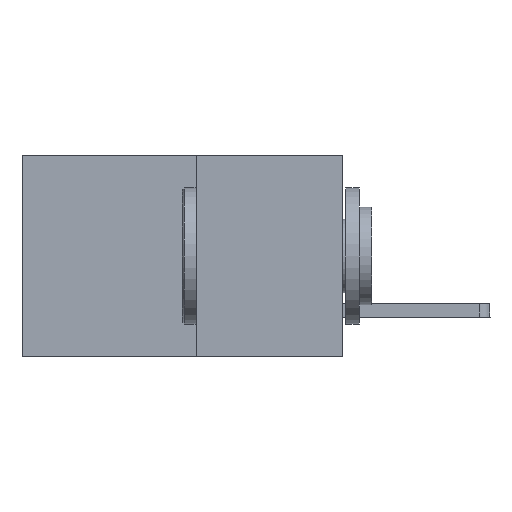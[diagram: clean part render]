
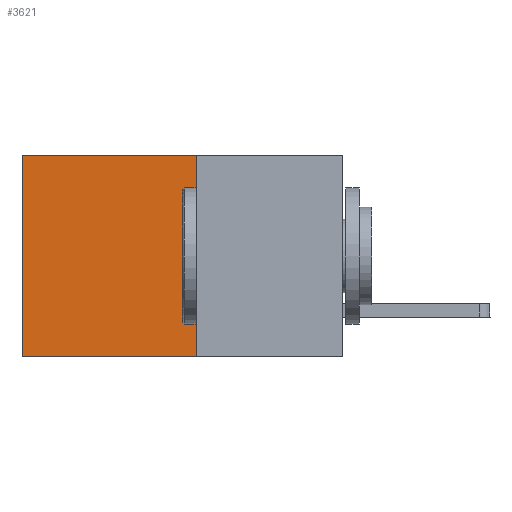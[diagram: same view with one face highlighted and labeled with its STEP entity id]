
A CAD part, left-side view. The second image highlights one B-rep face of the part: STEP entity #3621.
In plain terms, the highlighted planar face has unit normal (-1, 0, 0).
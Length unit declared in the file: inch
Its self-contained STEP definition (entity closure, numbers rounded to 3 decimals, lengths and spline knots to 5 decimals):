
#257 = AXIS2_PLACEMENT_3D ( 'NONE', #3014, #3923, #6539 ) ;
#1044 = DIRECTION ( 'NONE',  ( 0., 0., -1. ) ) ;
#1153 = LINE ( 'NONE', #7173, #1815 ) ;
#1399 = EDGE_CURVE ( 'NONE', #9571, #8217, #5571, .T. ) ;
#1629 = EDGE_LOOP ( 'NONE', ( #9456, #3275, #3218, #3060 ) ) ;
#1815 = VECTOR ( 'NONE', #8874, 39.37008 ) ;
#2356 = LINE ( 'NONE', #8494, #7103 ) ;
#3014 = CARTESIAN_POINT ( 'NONE',  ( 0.277, 0.27, -0.37 ) ) ;
#3038 = CARTESIAN_POINT ( 'NONE',  ( 0.277, 0.27, 0. ) ) ;
#3060 = ORIENTED_EDGE ( 'NONE', *, *, #9333, .T. ) ;
#3218 = ORIENTED_EDGE ( 'NONE', *, *, #3252, .F. ) ;
#3231 = VECTOR ( 'NONE', #1044, 39.37008 ) ;
#3252 = EDGE_CURVE ( 'NONE', #10536, #3387, #7200, .T. ) ;
#3275 = ORIENTED_EDGE ( 'NONE', *, *, #7054, .F. ) ;
#3387 = VERTEX_POINT ( 'NONE', #6623 ) ;
#3621 = ADVANCED_FACE ( 'NONE', ( #9146 ), #8353, .F. ) ;
#3761 = CARTESIAN_POINT ( 'NONE',  ( 0.277, 0.59, -0.37 ) ) ;
#3923 = DIRECTION ( 'NONE',  ( 1., 0., 0. ) ) ;
#3952 = DIRECTION ( 'NONE',  ( 0., 0., -1. ) ) ;
#4959 = VECTOR ( 'NONE', #3952, 39.37008 ) ;
#5571 = LINE ( 'NONE', #3761, #3231 ) ;
#6509 = DIRECTION ( 'NONE',  ( 0., 1., 0. ) ) ;
#6539 = DIRECTION ( 'NONE',  ( 0., 0., -1. ) ) ;
#6623 = CARTESIAN_POINT ( 'NONE',  ( 0.277, 0.27, -0.37 ) ) ;
#7054 = EDGE_CURVE ( 'NONE', #3387, #8217, #1153, .T. ) ;
#7103 = VECTOR ( 'NONE', #6509, 39.37008 ) ;
#7173 = CARTESIAN_POINT ( 'NONE',  ( 0.277, 0.27, -0.37 ) ) ;
#7200 = LINE ( 'NONE', #9811, #4959 ) ;
#8217 = VERTEX_POINT ( 'NONE', #11012 ) ;
#8353 = PLANE ( 'NONE',  #257 ) ;
#8494 = CARTESIAN_POINT ( 'NONE',  ( 0.277, 0.27, 0. ) ) ;
#8874 = DIRECTION ( 'NONE',  ( 0., 1., 0. ) ) ;
#9146 = FACE_OUTER_BOUND ( 'NONE', #1629, .T. ) ;
#9333 = EDGE_CURVE ( 'NONE', #10536, #9571, #2356, .T. ) ;
#9456 = ORIENTED_EDGE ( 'NONE', *, *, #1399, .T. ) ;
#9571 = VERTEX_POINT ( 'NONE', #10297 ) ;
#9811 = CARTESIAN_POINT ( 'NONE',  ( 0.277, 0.27, -0.37 ) ) ;
#10297 = CARTESIAN_POINT ( 'NONE',  ( 0.277, 0.59, 0. ) ) ;
#10536 = VERTEX_POINT ( 'NONE', #3038 ) ;
#11012 = CARTESIAN_POINT ( 'NONE',  ( 0.277, 0.59, -0.37 ) ) ;
